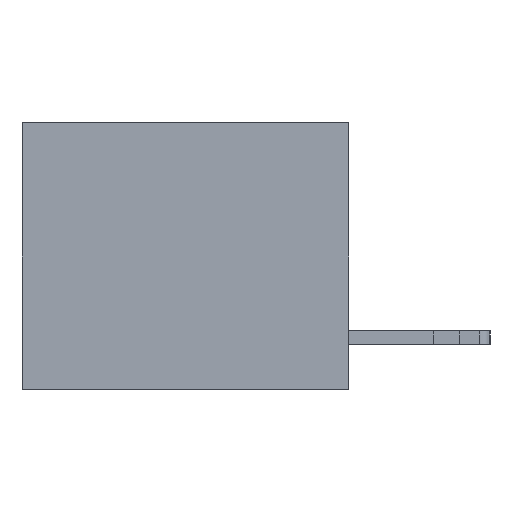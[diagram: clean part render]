
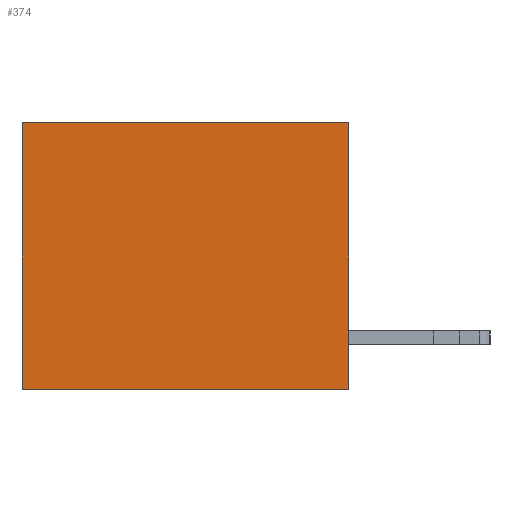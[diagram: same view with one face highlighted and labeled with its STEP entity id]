
A CAD part, left-side view. The second image highlights one B-rep face of the part: STEP entity #374.
In plain terms, the highlighted planar face has unit normal (-1, 0, 0).
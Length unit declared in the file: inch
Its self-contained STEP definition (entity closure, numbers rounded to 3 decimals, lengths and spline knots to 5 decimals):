
#271 = ORIENTED_EDGE ( 'NONE', *, *, #4754, .T. ) ;
#374 = ADVANCED_FACE ( 'NONE', ( #1305 ), #5831, .F. ) ;
#686 = DIRECTION ( 'NONE',  ( 0., 0., -1. ) ) ;
#1305 = FACE_OUTER_BOUND ( 'NONE', #14383, .T. ) ;
#1902 = DIRECTION ( 'NONE',  ( 0., 0., -1. ) ) ;
#2105 = CARTESIAN_POINT ( 'NONE',  ( 0.3165, 0., -0.49 ) ) ;
#2124 = LINE ( 'NONE', #12728, #5698 ) ;
#3051 = CARTESIAN_POINT ( 'NONE',  ( 0.3165, 0., -0.49 ) ) ;
#3214 = CARTESIAN_POINT ( 'NONE',  ( 0.3165, 0., 0. ) ) ;
#3408 = LINE ( 'NONE', #3214, #11173 ) ;
#3911 = VECTOR ( 'NONE', #8236, 39.37008 ) ;
#4754 = EDGE_CURVE ( 'NONE', #11191, #11435, #3408, .T. ) ;
#5698 = VECTOR ( 'NONE', #686, 39.37008 ) ;
#5707 = AXIS2_PLACEMENT_3D ( 'NONE', #3051, #10624, #1902 ) ;
#5831 = PLANE ( 'NONE',  #5707 ) ;
#6773 = EDGE_CURVE ( 'NONE', #12390, #8985, #7104, .T. ) ;
#7104 = LINE ( 'NONE', #8021, #3911 ) ;
#7858 = CARTESIAN_POINT ( 'NONE',  ( 0.3165, 0.6, -0.49 ) ) ;
#8021 = CARTESIAN_POINT ( 'NONE',  ( 0.3165, 0., -0.49 ) ) ;
#8236 = DIRECTION ( 'NONE',  ( 0., 1., 0. ) ) ;
#8387 = VECTOR ( 'NONE', #15437, 39.37008 ) ;
#8985 = VERTEX_POINT ( 'NONE', #7858 ) ;
#10452 = LINE ( 'NONE', #2105, #8387 ) ;
#10579 = ORIENTED_EDGE ( 'NONE', *, *, #12529, .F. ) ;
#10614 = ORIENTED_EDGE ( 'NONE', *, *, #13683, .T. ) ;
#10624 = DIRECTION ( 'NONE',  ( 1., 0., 0. ) ) ;
#11173 = VECTOR ( 'NONE', #12895, 39.37008 ) ;
#11191 = VERTEX_POINT ( 'NONE', #11465 ) ;
#11435 = VERTEX_POINT ( 'NONE', #15656 ) ;
#11465 = CARTESIAN_POINT ( 'NONE',  ( 0.3165, 0., 0. ) ) ;
#12390 = VERTEX_POINT ( 'NONE', #15343 ) ;
#12529 = EDGE_CURVE ( 'NONE', #11191, #12390, #10452, .T. ) ;
#12728 = CARTESIAN_POINT ( 'NONE',  ( 0.3165, 0.6, -0.49 ) ) ;
#12895 = DIRECTION ( 'NONE',  ( 0., 1., 0. ) ) ;
#13683 = EDGE_CURVE ( 'NONE', #11435, #8985, #2124, .T. ) ;
#14383 = EDGE_LOOP ( 'NONE', ( #10614, #15644, #10579, #271 ) ) ;
#15343 = CARTESIAN_POINT ( 'NONE',  ( 0.3165, 0., -0.49 ) ) ;
#15437 = DIRECTION ( 'NONE',  ( 0., 0., -1. ) ) ;
#15644 = ORIENTED_EDGE ( 'NONE', *, *, #6773, .F. ) ;
#15656 = CARTESIAN_POINT ( 'NONE',  ( 0.3165, 0.6, 0. ) ) ;
